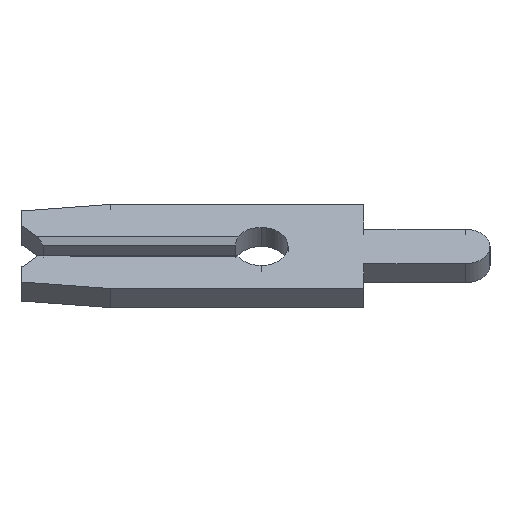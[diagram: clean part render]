
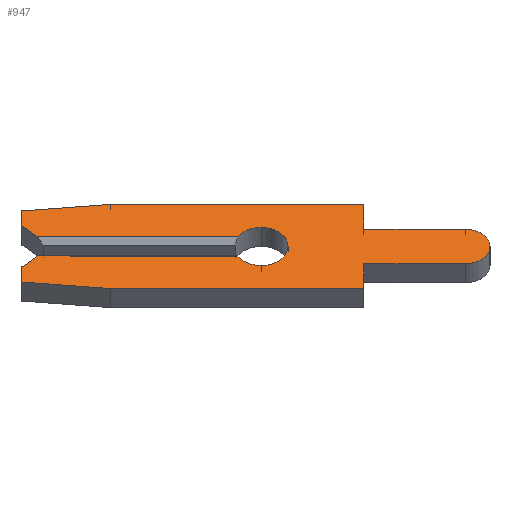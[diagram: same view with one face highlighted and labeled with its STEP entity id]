
A CAD part, left-side view. The second image highlights one B-rep face of the part: STEP entity #947.
In plain terms, the highlighted face is planar.
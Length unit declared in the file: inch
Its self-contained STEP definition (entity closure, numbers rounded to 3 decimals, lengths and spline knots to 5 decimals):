
#1 = LINE ( 'NONE', #265, #590 ) ;
#2 = CARTESIAN_POINT ( 'NONE',  ( -0.013, 0., -0.026 ) ) ;
#15 = VERTEX_POINT ( 'NONE', #826 ) ;
#17 = EDGE_CURVE ( 'NONE', #15, #467, #49, .T. ) ;
#22 = DIRECTION ( 'NONE',  ( 0., 0.995, 0.105 ) ) ;
#46 = FACE_OUTER_BOUND ( 'NONE', #351, .T. ) ;
#49 = LINE ( 'NONE', #1060, #1184 ) ;
#64 = AXIS2_PLACEMENT_3D ( 'NONE', #600, #1264, #474 ) ;
#77 = CARTESIAN_POINT ( 'NONE',  ( -0.013, 0.231, 0.013 ) ) ;
#85 = VECTOR ( 'NONE', #1205, 39.37008 ) ;
#106 = ORIENTED_EDGE ( 'NONE', *, *, #1072, .F. ) ;
#108 = VECTOR ( 'NONE', #1393, 39.37008 ) ;
#136 = VECTOR ( 'NONE', #380, 39.37008 ) ;
#137 = DIRECTION ( 'NONE',  ( 0., 0., -1. ) ) ;
#151 = VERTEX_POINT ( 'NONE', #1043 ) ;
#152 = ORIENTED_EDGE ( 'NONE', *, *, #17, .F. ) ;
#181 = DIRECTION ( 'NONE',  ( 0., 0., 1. ) ) ;
#189 = VERTEX_POINT ( 'NONE', #211 ) ;
#211 = CARTESIAN_POINT ( 'NONE',  ( -0.013, 0.231, 0.028 ) ) ;
#214 = VECTOR ( 'NONE', #22, 39.37008 ) ;
#231 = ORIENTED_EDGE ( 'NONE', *, *, #1284, .F. ) ;
#237 = LINE ( 'NONE', #1330, #252 ) ;
#252 = VECTOR ( 'NONE', #544, 39.37008 ) ;
#265 = CARTESIAN_POINT ( 'NONE',  ( -0.013, -0.099, -0.0235 ) ) ;
#275 = DIRECTION ( 'NONE',  ( -1., 0., 0. ) ) ;
#286 = VERTEX_POINT ( 'NONE', #1192 ) ;
#288 = CARTESIAN_POINT ( 'NONE',  ( -0.013, 0., 0.026 ) ) ;
#295 = ORIENTED_EDGE ( 'NONE', *, *, #810, .F. ) ;
#305 = ORIENTED_EDGE ( 'NONE', *, *, #935, .F. ) ;
#315 = LINE ( 'NONE', #1079, #85 ) ;
#327 = VERTEX_POINT ( 'NONE', #627 ) ;
#342 = DIRECTION ( 'NONE',  ( 0., 0., -1. ) ) ;
#350 = AXIS2_PLACEMENT_3D ( 'NONE', #628, #641, #857 ) ;
#351 = EDGE_LOOP ( 'NONE', ( #664, #295, #1282, #391, #497, #152, #106, #413, #1248, #1171, #305, #231, #431, #1340, #965, #972, #842, #1129 ) ) ;
#362 = PLANE ( 'NONE',  #64 ) ;
#373 = VERTEX_POINT ( 'NONE', #1222 ) ;
#380 = DIRECTION ( 'NONE',  ( 0., -1., 0. ) ) ;
#391 = ORIENTED_EDGE ( 'NONE', *, *, #961, .F. ) ;
#392 = VERTEX_POINT ( 'NONE', #987 ) ;
#394 = DIRECTION ( 'NONE',  ( 0., -0.707, 0.707 ) ) ;
#395 = LINE ( 'NONE', #1274, #108 ) ;
#413 = ORIENTED_EDGE ( 'NONE', *, *, #416, .F. ) ;
#414 = VECTOR ( 'NONE', #1296, 39.37008 ) ;
#416 = EDGE_CURVE ( 'NONE', #1265, #286, #866, .T. ) ;
#431 = ORIENTED_EDGE ( 'NONE', *, *, #524, .F. ) ;
#437 = AXIS2_PLACEMENT_3D ( 'NONE', #1255, #1368, #479 ) ;
#455 = CARTESIAN_POINT ( 'NONE',  ( -0.013, -0.099, 0.0575 ) ) ;
#460 = CARTESIAN_POINT ( 'NONE',  ( -0.013, 0., 0. ) ) ;
#467 = VERTEX_POINT ( 'NONE', #1102 ) ;
#474 = DIRECTION ( 'NONE',  ( 0., 0., -1. ) ) ;
#479 = DIRECTION ( 'NONE',  ( 0., 0., -1. ) ) ;
#497 = ORIENTED_EDGE ( 'NONE', *, *, #1009, .F. ) ;
#503 = CIRCLE ( 'NONE', #1331, 0.026 ) ;
#524 = EDGE_CURVE ( 'NONE', #151, #828, #1323, .T. ) ;
#525 = VECTOR ( 'NONE', #1128, 39.37008 ) ;
#544 = DIRECTION ( 'NONE',  ( 0., -0.995, 0.105 ) ) ;
#556 = VERTEX_POINT ( 'NONE', #2 ) ;
#572 = EDGE_CURVE ( 'NONE', #937, #946, #237, .T. ) ;
#586 = VERTEX_POINT ( 'NONE', #776 ) ;
#590 = VECTOR ( 'NONE', #929, 39.37008 ) ;
#600 = CARTESIAN_POINT ( 'NONE',  ( -0.013, 0., 0. ) ) ;
#609 = CARTESIAN_POINT ( 'NONE',  ( -0.013, 0.231, -0.028 ) ) ;
#627 = CARTESIAN_POINT ( 'NONE',  ( -0.013, -0.099, 0.0575 ) ) ;
#628 = CARTESIAN_POINT ( 'NONE',  ( -0.013, -0.1975, 0. ) ) ;
#641 = DIRECTION ( 'NONE',  ( 1., 0., 0. ) ) ;
#650 = DIRECTION ( 'NONE',  ( 0., -1., 0. ) ) ;
#664 = ORIENTED_EDGE ( 'NONE', *, *, #1062, .T. ) ;
#666 = LINE ( 'NONE', #455, #525 ) ;
#673 = EDGE_CURVE ( 'NONE', #556, #1001, #503, .T. ) ;
#687 = CARTESIAN_POINT ( 'NONE',  ( -0.013, -0.099, -0.0575 ) ) ;
#762 = CARTESIAN_POINT ( 'NONE',  ( -0.013, 0.146, -0.0575 ) ) ;
#767 = EDGE_CURVE ( 'NONE', #327, #151, #666, .T. ) ;
#776 = CARTESIAN_POINT ( 'NONE',  ( -0.013, 0.02252, -0.013 ) ) ;
#782 = AXIS2_PLACEMENT_3D ( 'NONE', #1250, #275, #137 ) ;
#789 = DIRECTION ( 'NONE',  ( -1., 0., 0. ) ) ;
#797 = VERTEX_POINT ( 'NONE', #687 ) ;
#806 = VERTEX_POINT ( 'NONE', #1351 ) ;
#807 = DIRECTION ( 'NONE',  ( 0., 1., 0. ) ) ;
#810 = EDGE_CURVE ( 'NONE', #1001, #806, #1019, .T. ) ;
#824 = CIRCLE ( 'NONE', #437, 0.026 ) ;
#826 = CARTESIAN_POINT ( 'NONE',  ( -0.013, 0.231, -0.028 ) ) ;
#828 = VERTEX_POINT ( 'NONE', #1008 ) ;
#832 = CARTESIAN_POINT ( 'NONE',  ( -0.013, 0., -0.013 ) ) ;
#842 = ORIENTED_EDGE ( 'NONE', *, *, #1036, .F. ) ;
#846 = CARTESIAN_POINT ( 'NONE',  ( -0.013, 0.146, 0.0575 ) ) ;
#855 = CARTESIAN_POINT ( 'NONE',  ( -0.013, 0.216, 0.013 ) ) ;
#857 = DIRECTION ( 'NONE',  ( 0., 0., 1. ) ) ;
#866 = LINE ( 'NONE', #1108, #214 ) ;
#899 = LINE ( 'NONE', #846, #1413 ) ;
#905 = EDGE_CURVE ( 'NONE', #797, #1265, #915, .T. ) ;
#915 = LINE ( 'NONE', #1364, #1160 ) ;
#929 = DIRECTION ( 'NONE',  ( 0., 1., 0. ) ) ;
#935 = EDGE_CURVE ( 'NONE', #392, #373, #1, .T. ) ;
#937 = VERTEX_POINT ( 'NONE', #1152 ) ;
#946 = VERTEX_POINT ( 'NONE', #1148 ) ;
#947 = ADVANCED_FACE ( 'NONE', ( #46 ), #362, .F. ) ;
#961 = EDGE_CURVE ( 'NONE', #586, #556, #824, .T. ) ;
#965 = ORIENTED_EDGE ( 'NONE', *, *, #1387, .F. ) ;
#967 = LINE ( 'NONE', #832, #1018 ) ;
#972 = ORIENTED_EDGE ( 'NONE', *, *, #572, .F. ) ;
#987 = CARTESIAN_POINT ( 'NONE',  ( -0.013, -0.1975, -0.0235 ) ) ;
#989 = VECTOR ( 'NONE', #1203, 39.37008 ) ;
#1001 = VERTEX_POINT ( 'NONE', #288 ) ;
#1004 = VECTOR ( 'NONE', #181, 39.37008 ) ;
#1008 = CARTESIAN_POINT ( 'NONE',  ( -0.013, -0.1975, 0.0235 ) ) ;
#1009 = EDGE_CURVE ( 'NONE', #467, #586, #967, .T. ) ;
#1018 = VECTOR ( 'NONE', #1157, 39.37008 ) ;
#1019 = CIRCLE ( 'NONE', #782, 0.026 ) ;
#1036 = EDGE_CURVE ( 'NONE', #189, #937, #1215, .T. ) ;
#1043 = CARTESIAN_POINT ( 'NONE',  ( -0.013, -0.099, 0.0235 ) ) ;
#1060 = CARTESIAN_POINT ( 'NONE',  ( -0.013, 0.2105, -0.0075 ) ) ;
#1061 = LINE ( 'NONE', #77, #136 ) ;
#1062 = EDGE_CURVE ( 'NONE', #1228, #806, #1061, .T. ) ;
#1072 = EDGE_CURVE ( 'NONE', #286, #15, #1269, .T. ) ;
#1079 = CARTESIAN_POINT ( 'NONE',  ( -0.013, 0.2105, 0.0075 ) ) ;
#1102 = CARTESIAN_POINT ( 'NONE',  ( -0.013, 0.216, -0.013 ) ) ;
#1108 = CARTESIAN_POINT ( 'NONE',  ( -0.013, 0.231, -0.04857 ) ) ;
#1128 = DIRECTION ( 'NONE',  ( 0., 0., -1. ) ) ;
#1129 = ORIENTED_EDGE ( 'NONE', *, *, #1239, .F. ) ;
#1135 = EDGE_CURVE ( 'NONE', #373, #797, #395, .T. ) ;
#1148 = CARTESIAN_POINT ( 'NONE',  ( -0.013, 0.146, 0.0575 ) ) ;
#1152 = CARTESIAN_POINT ( 'NONE',  ( -0.013, 0.231, 0.04857 ) ) ;
#1157 = DIRECTION ( 'NONE',  ( 0., -1., 0. ) ) ;
#1160 = VECTOR ( 'NONE', #807, 39.37008 ) ;
#1164 = CARTESIAN_POINT ( 'NONE',  ( -0.013, 0.231, 0.028 ) ) ;
#1171 = ORIENTED_EDGE ( 'NONE', *, *, #1135, .F. ) ;
#1184 = VECTOR ( 'NONE', #394, 39.37008 ) ;
#1192 = CARTESIAN_POINT ( 'NONE',  ( -0.013, 0.231, -0.04857 ) ) ;
#1203 = DIRECTION ( 'NONE',  ( 0., -1., 0. ) ) ;
#1205 = DIRECTION ( 'NONE',  ( 0., 0.707, 0.707 ) ) ;
#1215 = LINE ( 'NONE', #1164, #414 ) ;
#1222 = CARTESIAN_POINT ( 'NONE',  ( -0.013, -0.099, -0.0235 ) ) ;
#1228 = VERTEX_POINT ( 'NONE', #855 ) ;
#1232 = CIRCLE ( 'NONE', #350, 0.0235 ) ;
#1239 = EDGE_CURVE ( 'NONE', #1228, #189, #315, .T. ) ;
#1248 = ORIENTED_EDGE ( 'NONE', *, *, #905, .F. ) ;
#1250 = CARTESIAN_POINT ( 'NONE',  ( -0.013, 0., 0. ) ) ;
#1255 = CARTESIAN_POINT ( 'NONE',  ( -0.013, 0., 0. ) ) ;
#1264 = DIRECTION ( 'NONE',  ( 1., 0., 0. ) ) ;
#1265 = VERTEX_POINT ( 'NONE', #762 ) ;
#1269 = LINE ( 'NONE', #609, #1004 ) ;
#1274 = CARTESIAN_POINT ( 'NONE',  ( -0.013, -0.099, -0.0575 ) ) ;
#1282 = ORIENTED_EDGE ( 'NONE', *, *, #673, .F. ) ;
#1284 = EDGE_CURVE ( 'NONE', #828, #392, #1232, .T. ) ;
#1296 = DIRECTION ( 'NONE',  ( 0., 0., 1. ) ) ;
#1323 = LINE ( 'NONE', #1326, #989 ) ;
#1326 = CARTESIAN_POINT ( 'NONE',  ( -0.013, -0.099, 0.0235 ) ) ;
#1330 = CARTESIAN_POINT ( 'NONE',  ( -0.013, 0.231, 0.04857 ) ) ;
#1331 = AXIS2_PLACEMENT_3D ( 'NONE', #460, #789, #342 ) ;
#1340 = ORIENTED_EDGE ( 'NONE', *, *, #767, .F. ) ;
#1351 = CARTESIAN_POINT ( 'NONE',  ( -0.013, 0.02252, 0.013 ) ) ;
#1364 = CARTESIAN_POINT ( 'NONE',  ( -0.013, 0.146, -0.0575 ) ) ;
#1368 = DIRECTION ( 'NONE',  ( -1., 0., 0. ) ) ;
#1387 = EDGE_CURVE ( 'NONE', #946, #327, #899, .T. ) ;
#1393 = DIRECTION ( 'NONE',  ( 0., 0., -1. ) ) ;
#1413 = VECTOR ( 'NONE', #650, 39.37008 ) ;
